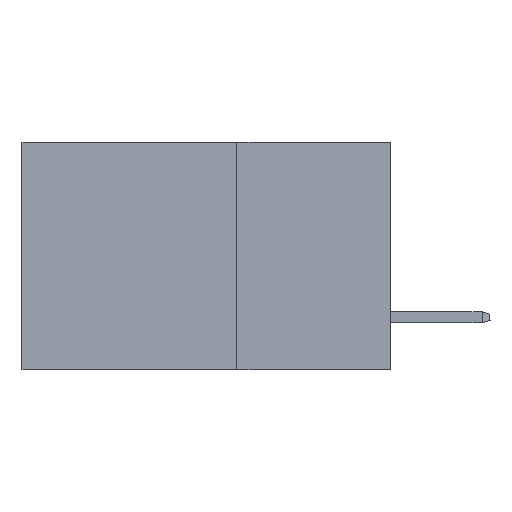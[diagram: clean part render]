
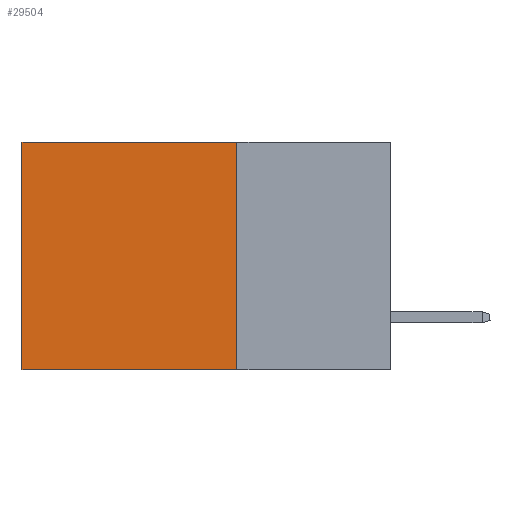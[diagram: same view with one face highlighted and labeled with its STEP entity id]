
A CAD part, left-side view. The second image highlights one B-rep face of the part: STEP entity #29504.
In plain terms, the highlighted planar face has unit normal (-1, 0, 0).
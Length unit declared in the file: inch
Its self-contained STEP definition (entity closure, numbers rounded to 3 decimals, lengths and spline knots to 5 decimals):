
#381 = VECTOR ( 'NONE', #11691, 39.37008 ) ;
#479 = LINE ( 'NONE', #9102, #24721 ) ;
#640 = VERTEX_POINT ( 'NONE', #26915 ) ;
#2036 = CARTESIAN_POINT ( 'NONE',  ( 0.2875, 0.6, -0.37 ) ) ;
#2270 = EDGE_CURVE ( 'NONE', #640, #7222, #29038, .T. ) ;
#2529 = CARTESIAN_POINT ( 'NONE',  ( 0.2875, 0.25, 0. ) ) ;
#3198 = ORIENTED_EDGE ( 'NONE', *, *, #25917, .T. ) ;
#3910 = LINE ( 'NONE', #2529, #28151 ) ;
#4343 = ORIENTED_EDGE ( 'NONE', *, *, #2270, .F. ) ;
#5630 = VERTEX_POINT ( 'NONE', #25850 ) ;
#6316 = DIRECTION ( 'NONE',  ( 1., 0., 0. ) ) ;
#6900 = DIRECTION ( 'NONE',  ( 0., 0., -1. ) ) ;
#7222 = VERTEX_POINT ( 'NONE', #2036 ) ;
#8959 = FACE_OUTER_BOUND ( 'NONE', #24093, .T. ) ;
#9032 = CARTESIAN_POINT ( 'NONE',  ( 0.2875, 0.25, -0.37 ) ) ;
#9102 = CARTESIAN_POINT ( 'NONE',  ( 0.2875, 0.25, 0. ) ) ;
#11691 = DIRECTION ( 'NONE',  ( 0., 1., 0. ) ) ;
#11966 = ORIENTED_EDGE ( 'NONE', *, *, #24742, .T. ) ;
#12317 = VECTOR ( 'NONE', #6900, 39.37008 ) ;
#17577 = DIRECTION ( 'NONE',  ( 0., 0., -1. ) ) ;
#18635 = VERTEX_POINT ( 'NONE', #25427 ) ;
#20482 = CARTESIAN_POINT ( 'NONE',  ( 0.2875, 0.25, 0. ) ) ;
#20514 = AXIS2_PLACEMENT_3D ( 'NONE', #20482, #6316, #25361 ) ;
#22922 = PLANE ( 'NONE',  #20514 ) ;
#22928 = DIRECTION ( 'NONE',  ( 0., 1., 0. ) ) ;
#23199 = CARTESIAN_POINT ( 'NONE',  ( 0.2875, 0.6, 0. ) ) ;
#24066 = ORIENTED_EDGE ( 'NONE', *, *, #27837, .F. ) ;
#24093 = EDGE_LOOP ( 'NONE', ( #11966, #4343, #24066, #3198 ) ) ;
#24721 = VECTOR ( 'NONE', #22928, 39.37008 ) ;
#24742 = EDGE_CURVE ( 'NONE', #18635, #7222, #24779, .T. ) ;
#24779 = LINE ( 'NONE', #23199, #12317 ) ;
#25361 = DIRECTION ( 'NONE',  ( 0., 0., -1. ) ) ;
#25427 = CARTESIAN_POINT ( 'NONE',  ( 0.2875, 0.6, 0. ) ) ;
#25850 = CARTESIAN_POINT ( 'NONE',  ( 0.2875, 0.25, 0. ) ) ;
#25917 = EDGE_CURVE ( 'NONE', #5630, #18635, #479, .T. ) ;
#26915 = CARTESIAN_POINT ( 'NONE',  ( 0.2875, 0.25, -0.37 ) ) ;
#27837 = EDGE_CURVE ( 'NONE', #5630, #640, #3910, .T. ) ;
#28151 = VECTOR ( 'NONE', #17577, 39.37008 ) ;
#29038 = LINE ( 'NONE', #9032, #381 ) ;
#29504 = ADVANCED_FACE ( 'NONE', ( #8959 ), #22922, .F. ) ;
